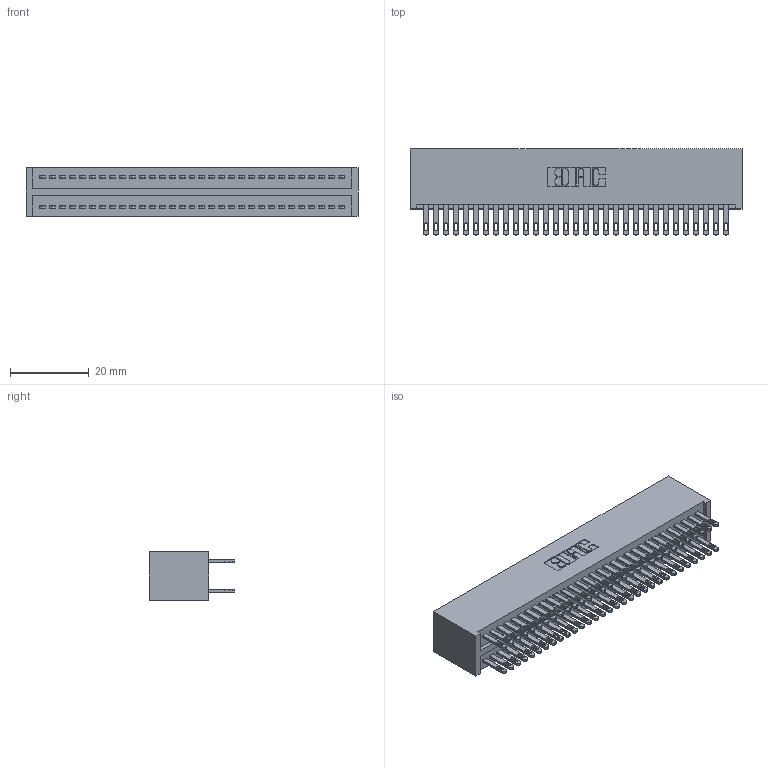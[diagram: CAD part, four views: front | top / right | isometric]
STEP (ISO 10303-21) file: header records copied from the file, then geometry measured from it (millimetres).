
FILE_DESCRIPTION (( 'STEP AP203' ), '1' );
FILE_NAME ('325-062-500-201.STEP', '2020-02-25T02:54:02', ( '' ), ( '' ), 'SwSTEP 2.0', 'SolidWorks 2016', '' );
FILE_SCHEMA (( 'CONFIG_CONTROL_DESIGN' ));
Length unit declared in the file: inch
Products named in the file (3): 325-292-001_325-293-100; 325 Part_Lugless; 325-062-500-201
Assembly tree (63 placements, depth 2):
  325-062-500-201
    325 Part_Lugless
    325-292-001_325-293-100  x62
Bounding box: 84.38 x 21.84 x 12.45 mm (x, y, z)
Volume: 11589.9 mm3; surface area: 15076.4 mm2
Topology: 63 solids, 63 shells, 3082 faces, 9401 edges, 6266 vertices
Faces by surface type: plane 1926, cylinder 1156
Entity records: 21019 total; most frequent: CARTESIAN_POINT 3494, ORIENTED_EDGE 3430, DIRECTION 2999, EDGE_CURVE 1715, LINE 1591, VECTOR 1591, VERTEX_POINT 1142, AXIS2_PLACEMENT_3D 704
